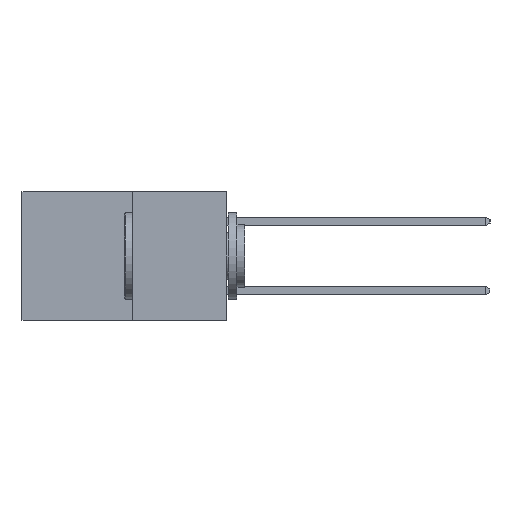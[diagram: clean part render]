
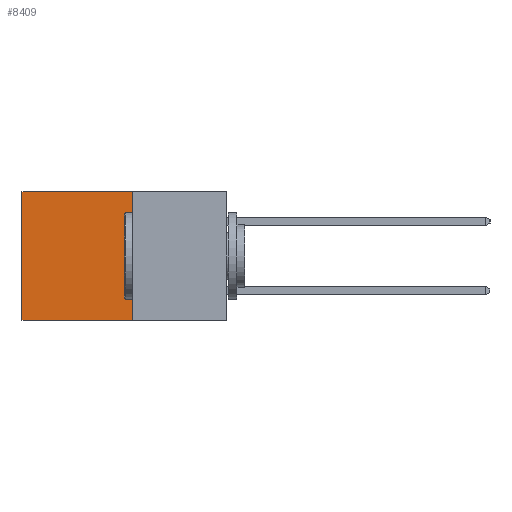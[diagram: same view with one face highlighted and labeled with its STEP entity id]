
A CAD part, left-side view. The second image highlights one B-rep face of the part: STEP entity #8409.
In plain terms, the highlighted planar face has unit normal (-1, 0, 0).
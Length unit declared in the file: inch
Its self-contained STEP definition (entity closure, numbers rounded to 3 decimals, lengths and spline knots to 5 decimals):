
#179 = VECTOR ( 'NONE', #8318, 39.37008 ) ;
#419 = PLANE ( 'NONE',  #10600 ) ;
#712 = CARTESIAN_POINT ( 'NONE',  ( 0.277, 0.27, 0. ) ) ;
#1007 = CARTESIAN_POINT ( 'NONE',  ( 0.277, 0.27, 0. ) ) ;
#1931 = DIRECTION ( 'NONE',  ( 0., 1., 0. ) ) ;
#1933 = LINE ( 'NONE', #6290, #6182 ) ;
#2024 = ORIENTED_EDGE ( 'NONE', *, *, #10485, .T. ) ;
#2292 = DIRECTION ( 'NONE',  ( 0., 0., -1. ) ) ;
#2847 = ORIENTED_EDGE ( 'NONE', *, *, #9026, .F. ) ;
#2904 = LINE ( 'NONE', #8101, #179 ) ;
#2926 = VERTEX_POINT ( 'NONE', #712 ) ;
#2954 = CARTESIAN_POINT ( 'NONE',  ( 0.277, 0.59, 0. ) ) ;
#3084 = CARTESIAN_POINT ( 'NONE',  ( 0.277, 0.59, -0.37 ) ) ;
#3381 = ORIENTED_EDGE ( 'NONE', *, *, #3904, .F. ) ;
#3757 = VERTEX_POINT ( 'NONE', #10897 ) ;
#3904 = EDGE_CURVE ( 'NONE', #2926, #7809, #2904, .T. ) ;
#4098 = ORIENTED_EDGE ( 'NONE', *, *, #7193, .T. ) ;
#4457 = VECTOR ( 'NONE', #5596, 39.37008 ) ;
#4540 = VECTOR ( 'NONE', #1931, 39.37008 ) ;
#4686 = EDGE_LOOP ( 'NONE', ( #2024, #2847, #3381, #4098 ) ) ;
#5283 = FACE_OUTER_BOUND ( 'NONE', #4686, .T. ) ;
#5596 = DIRECTION ( 'NONE',  ( 0., 0., -1. ) ) ;
#6182 = VECTOR ( 'NONE', #8897, 39.37008 ) ;
#6290 = CARTESIAN_POINT ( 'NONE',  ( 0.277, 0.27, -0.37 ) ) ;
#6485 = CARTESIAN_POINT ( 'NONE',  ( 0.277, 0.27, -0.37 ) ) ;
#6513 = LINE ( 'NONE', #1007, #4540 ) ;
#6701 = LINE ( 'NONE', #3084, #4457 ) ;
#7193 = EDGE_CURVE ( 'NONE', #2926, #7329, #6513, .T. ) ;
#7329 = VERTEX_POINT ( 'NONE', #2954 ) ;
#7358 = DIRECTION ( 'NONE',  ( 1., 0., 0. ) ) ;
#7809 = VERTEX_POINT ( 'NONE', #8513 ) ;
#8101 = CARTESIAN_POINT ( 'NONE',  ( 0.277, 0.27, -0.37 ) ) ;
#8318 = DIRECTION ( 'NONE',  ( 0., 0., -1. ) ) ;
#8409 = ADVANCED_FACE ( 'NONE', ( #5283 ), #419, .F. ) ;
#8513 = CARTESIAN_POINT ( 'NONE',  ( 0.277, 0.27, -0.37 ) ) ;
#8897 = DIRECTION ( 'NONE',  ( 0., 1., 0. ) ) ;
#9026 = EDGE_CURVE ( 'NONE', #7809, #3757, #1933, .T. ) ;
#10485 = EDGE_CURVE ( 'NONE', #7329, #3757, #6701, .T. ) ;
#10600 = AXIS2_PLACEMENT_3D ( 'NONE', #6485, #7358, #2292 ) ;
#10897 = CARTESIAN_POINT ( 'NONE',  ( 0.277, 0.59, -0.37 ) ) ;
